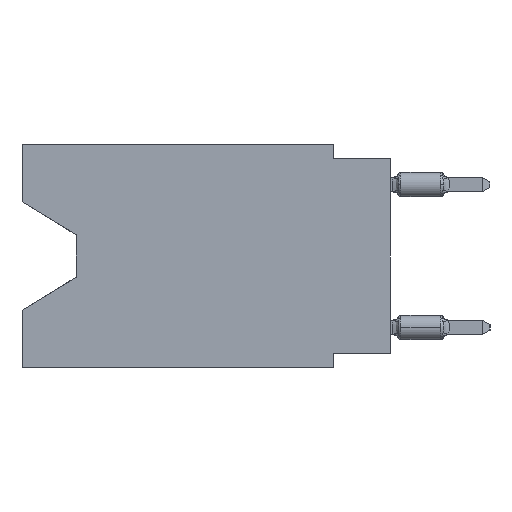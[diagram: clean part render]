
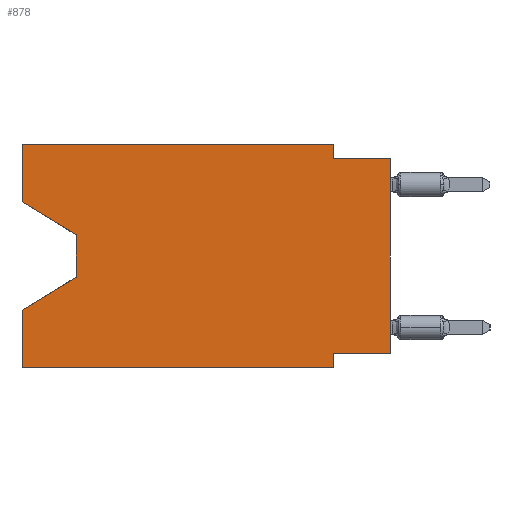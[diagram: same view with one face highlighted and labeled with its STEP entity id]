
A CAD part, left-side view. The second image highlights one B-rep face of the part: STEP entity #878.
In plain terms, the highlighted planar face has unit normal (-1, 0, 0).
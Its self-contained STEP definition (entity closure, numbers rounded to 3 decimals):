
#789 = VECTOR ( 'NONE', #22352, 1000. ) ;
#878 = ADVANCED_FACE ( 'NONE', ( #17411 ), #4393, .F. ) ;
#1516 = VECTOR ( 'NONE', #6726, 1000. ) ;
#1775 = VECTOR ( 'NONE', #4477, 1000. ) ;
#2033 = LINE ( 'NONE', #17337, #48750 ) ;
#3045 = DIRECTION ( 'NONE',  ( 0., 0.855, -0.519 ) ) ;
#3612 = VERTEX_POINT ( 'NONE', #25825 ) ;
#3628 = DIRECTION ( 'NONE',  ( 0., -0.855, -0.519 ) ) ;
#3823 = AXIS2_PLACEMENT_3D ( 'NONE', #45868, #45605, #33426 ) ;
#4393 = PLANE ( 'NONE',  #3823 ) ;
#4477 = DIRECTION ( 'NONE',  ( 0., 0., -1. ) ) ;
#4791 = EDGE_LOOP ( 'NONE', ( #31354, #34666, #33021, #26521, #33067, #46825, #30929, #9494, #25971, #29169, #30774, #31768 ) ) ;
#6206 = EDGE_CURVE ( 'NONE', #51415, #3612, #50116, .T. ) ;
#6726 = DIRECTION ( 'NONE',  ( 0., 0., -1. ) ) ;
#7189 = LINE ( 'NONE', #28363, #14545 ) ;
#7512 = DIRECTION ( 'NONE',  ( 0., 0., 1. ) ) ;
#8656 = CARTESIAN_POINT ( 'NONE',  ( 0., 2.54, -0.635 ) ) ;
#8818 = LINE ( 'NONE', #29183, #1775 ) ;
#9494 = ORIENTED_EDGE ( 'NONE', *, *, #18579, .T. ) ;
#10147 = VERTEX_POINT ( 'NONE', #53309 ) ;
#10259 = CARTESIAN_POINT ( 'NONE',  ( 0., 13.97, -4.013 ) ) ;
#11300 = CARTESIAN_POINT ( 'NONE',  ( 0., 16.383, 0. ) ) ;
#13036 = VERTEX_POINT ( 'NONE', #16094 ) ;
#13907 = CARTESIAN_POINT ( 'NONE',  ( 0., 0., -9.271 ) ) ;
#13978 = EDGE_CURVE ( 'NONE', #10147, #13036, #43870, .T. ) ;
#14545 = VECTOR ( 'NONE', #40284, 1000. ) ;
#14595 = EDGE_CURVE ( 'NONE', #38786, #28385, #7189, .T. ) ;
#14786 = CARTESIAN_POINT ( 'NONE',  ( 0., 16.383, -9.906 ) ) ;
#15407 = EDGE_CURVE ( 'NONE', #22776, #31989, #53095, .T. ) ;
#16094 = CARTESIAN_POINT ( 'NONE',  ( 0., 13.97, -5.893 ) ) ;
#16721 = LINE ( 'NONE', #44655, #47754 ) ;
#17254 = EDGE_CURVE ( 'NONE', #32202, #22776, #8818, .T. ) ;
#17337 = CARTESIAN_POINT ( 'NONE',  ( 0., 2.54, -9.906 ) ) ;
#17411 = FACE_OUTER_BOUND ( 'NONE', #4791, .T. ) ;
#18422 = EDGE_CURVE ( 'NONE', #3612, #32202, #22997, .T. ) ;
#18579 = EDGE_CURVE ( 'NONE', #23004, #31989, #16721, .T. ) ;
#20068 = VECTOR ( 'NONE', #27875, 1000. ) ;
#20586 = EDGE_CURVE ( 'NONE', #13036, #28385, #48605, .T. ) ;
#22352 = DIRECTION ( 'NONE',  ( 0., 1., 0. ) ) ;
#22776 = VERTEX_POINT ( 'NONE', #8656 ) ;
#22997 = LINE ( 'NONE', #11300, #20068 ) ;
#23004 = VERTEX_POINT ( 'NONE', #48722 ) ;
#23832 = CARTESIAN_POINT ( 'NONE',  ( 0., 0., -0.635 ) ) ;
#24553 = EDGE_CURVE ( 'NONE', #35388, #26805, #2033, .T. ) ;
#25085 = CARTESIAN_POINT ( 'NONE',  ( 0., 2.54, -9.906 ) ) ;
#25825 = CARTESIAN_POINT ( 'NONE',  ( 0., 16.383, 0. ) ) ;
#25971 = ORIENTED_EDGE ( 'NONE', *, *, #15407, .F. ) ;
#26475 = CARTESIAN_POINT ( 'NONE',  ( 0., 16.383, -7.36 ) ) ;
#26521 = ORIENTED_EDGE ( 'NONE', *, *, #14595, .F. ) ;
#26805 = VERTEX_POINT ( 'NONE', #25085 ) ;
#27875 = DIRECTION ( 'NONE',  ( 0., -1., 0. ) ) ;
#28363 = CARTESIAN_POINT ( 'NONE',  ( 0., 16.383, 0. ) ) ;
#28385 = VERTEX_POINT ( 'NONE', #26475 ) ;
#28605 = CARTESIAN_POINT ( 'NONE',  ( 0., 16.383, -2.546 ) ) ;
#28708 = VECTOR ( 'NONE', #40561, 1000. ) ;
#29169 = ORIENTED_EDGE ( 'NONE', *, *, #17254, .F. ) ;
#29183 = CARTESIAN_POINT ( 'NONE',  ( 0., 2.54, 0. ) ) ;
#29776 = CARTESIAN_POINT ( 'NONE',  ( 0., 2.54, 0. ) ) ;
#29784 = CARTESIAN_POINT ( 'NONE',  ( 0., 16.383, 0. ) ) ;
#30774 = ORIENTED_EDGE ( 'NONE', *, *, #18422, .F. ) ;
#30929 = ORIENTED_EDGE ( 'NONE', *, *, #45173, .F. ) ;
#31354 = ORIENTED_EDGE ( 'NONE', *, *, #39271, .T. ) ;
#31768 = ORIENTED_EDGE ( 'NONE', *, *, #6206, .F. ) ;
#31989 = VERTEX_POINT ( 'NONE', #46890 ) ;
#32202 = VERTEX_POINT ( 'NONE', #29776 ) ;
#32854 = VECTOR ( 'NONE', #40633, 1000. ) ;
#33021 = ORIENTED_EDGE ( 'NONE', *, *, #20586, .T. ) ;
#33067 = ORIENTED_EDGE ( 'NONE', *, *, #47817, .T. ) ;
#33426 = DIRECTION ( 'NONE',  ( 0., 0., -1. ) ) ;
#34666 = ORIENTED_EDGE ( 'NONE', *, *, #13978, .T. ) ;
#35144 = DIRECTION ( 'NONE',  ( 0., 0., -1. ) ) ;
#35388 = VERTEX_POINT ( 'NONE', #35453 ) ;
#35453 = CARTESIAN_POINT ( 'NONE',  ( 0., 2.54, -9.271 ) ) ;
#35602 = LINE ( 'NONE', #13907, #789 ) ;
#38786 = VERTEX_POINT ( 'NONE', #47393 ) ;
#39271 = EDGE_CURVE ( 'NONE', #51415, #10147, #40795, .T. ) ;
#40284 = DIRECTION ( 'NONE',  ( 0., 0., 1. ) ) ;
#40561 = DIRECTION ( 'NONE',  ( 0., -1., 0. ) ) ;
#40633 = DIRECTION ( 'NONE',  ( 0., -1., 0. ) ) ;
#40795 = LINE ( 'NONE', #28605, #49835 ) ;
#41741 = VECTOR ( 'NONE', #3045, 1000. ) ;
#42245 = DIRECTION ( 'NONE',  ( 0., 0., 1. ) ) ;
#43803 = LINE ( 'NONE', #14786, #28708 ) ;
#43870 = LINE ( 'NONE', #10259, #1516 ) ;
#44106 = CARTESIAN_POINT ( 'NONE',  ( 0., 16.383, -2.546 ) ) ;
#44531 = CARTESIAN_POINT ( 'NONE',  ( 0., 13.97, -5.893 ) ) ;
#44655 = CARTESIAN_POINT ( 'NONE',  ( 0., 0., 0. ) ) ;
#44814 = VECTOR ( 'NONE', #42245, 1000. ) ;
#45173 = EDGE_CURVE ( 'NONE', #23004, #35388, #35602, .T. ) ;
#45605 = DIRECTION ( 'NONE',  ( 1., 0., 0. ) ) ;
#45868 = CARTESIAN_POINT ( 'NONE',  ( 0., 16.383, 0. ) ) ;
#46825 = ORIENTED_EDGE ( 'NONE', *, *, #24553, .F. ) ;
#46890 = CARTESIAN_POINT ( 'NONE',  ( 0., 0., -0.635 ) ) ;
#47393 = CARTESIAN_POINT ( 'NONE',  ( 0., 16.383, -9.906 ) ) ;
#47754 = VECTOR ( 'NONE', #7512, 1000. ) ;
#47817 = EDGE_CURVE ( 'NONE', #38786, #26805, #43803, .T. ) ;
#48605 = LINE ( 'NONE', #44531, #41741 ) ;
#48722 = CARTESIAN_POINT ( 'NONE',  ( 0., 0., -9.271 ) ) ;
#48750 = VECTOR ( 'NONE', #35144, 1000. ) ;
#49835 = VECTOR ( 'NONE', #3628, 1000. ) ;
#50116 = LINE ( 'NONE', #29784, #44814 ) ;
#51415 = VERTEX_POINT ( 'NONE', #44106 ) ;
#53095 = LINE ( 'NONE', #23832, #32854 ) ;
#53309 = CARTESIAN_POINT ( 'NONE',  ( 0., 13.97, -4.013 ) ) ;
